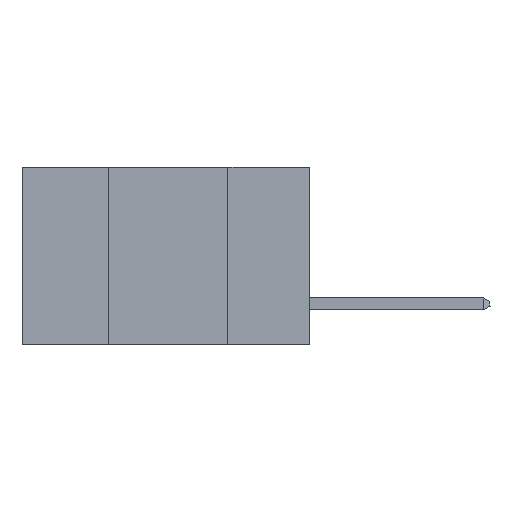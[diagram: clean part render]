
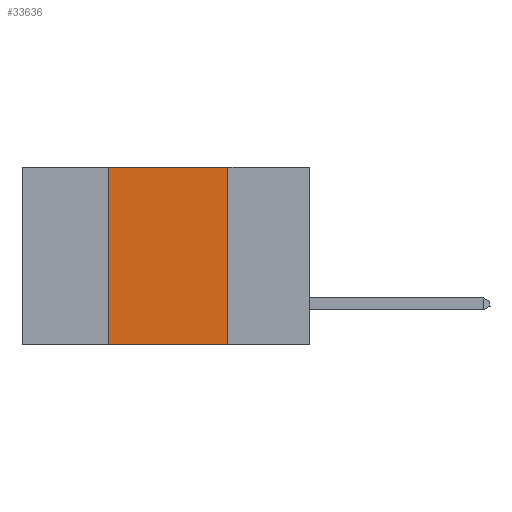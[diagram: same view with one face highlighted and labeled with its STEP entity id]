
A CAD part, left-side view. The second image highlights one B-rep face of the part: STEP entity #33636.
In plain terms, the highlighted planar face has unit normal (-1, 0, 0).
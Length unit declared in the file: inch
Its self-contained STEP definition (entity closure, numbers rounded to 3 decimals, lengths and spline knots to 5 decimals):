
#417 = ORIENTED_EDGE ( 'NONE', *, *, #23287, .F. ) ;
#500 = EDGE_CURVE ( 'NONE', #6923, #35511, #14397, .T. ) ;
#2125 = CARTESIAN_POINT ( 'NONE',  ( 0., 0.6, 0. ) ) ;
#2454 = VERTEX_POINT ( 'NONE', #45039 ) ;
#3004 = EDGE_LOOP ( 'NONE', ( #417, #21141, #40654, #37563 ) ) ;
#6719 = EDGE_CURVE ( 'NONE', #6923, #34437, #26632, .T. ) ;
#6923 = VERTEX_POINT ( 'NONE', #41657 ) ;
#8187 = CARTESIAN_POINT ( 'NONE',  ( 0., 0.6, -0.37 ) ) ;
#9260 = DIRECTION ( 'NONE',  ( 1., 0., 0. ) ) ;
#12655 = CARTESIAN_POINT ( 'NONE',  ( 0., 0.42, 0. ) ) ;
#13106 = DIRECTION ( 'NONE',  ( 0., 0., -1. ) ) ;
#13385 = FACE_OUTER_BOUND ( 'NONE', #3004, .T. ) ;
#14397 = LINE ( 'NONE', #8187, #44097 ) ;
#16595 = PLANE ( 'NONE',  #24044 ) ;
#16875 = EDGE_CURVE ( 'NONE', #34437, #2454, #33402, .T. ) ;
#20371 = CARTESIAN_POINT ( 'NONE',  ( 0., 0.17, 0. ) ) ;
#21027 = DIRECTION ( 'NONE',  ( 0., 0., -1. ) ) ;
#21141 = ORIENTED_EDGE ( 'NONE', *, *, #16875, .F. ) ;
#22989 = DIRECTION ( 'NONE',  ( 0., -1., 0. ) ) ;
#23287 = EDGE_CURVE ( 'NONE', #2454, #35511, #37252, .T. ) ;
#24044 = AXIS2_PLACEMENT_3D ( 'NONE', #2125, #9260, #13106 ) ;
#26156 = CARTESIAN_POINT ( 'NONE',  ( 0., 0.17, -0.37 ) ) ;
#26632 = LINE ( 'NONE', #39407, #32417 ) ;
#26880 = DIRECTION ( 'NONE',  ( 0., -1., 0. ) ) ;
#30858 = CARTESIAN_POINT ( 'NONE',  ( 0., 0.6, 0. ) ) ;
#32195 = DIRECTION ( 'NONE',  ( 0., 0., 1. ) ) ;
#32315 = VECTOR ( 'NONE', #26880, 39.37008 ) ;
#32417 = VECTOR ( 'NONE', #32195, 39.37008 ) ;
#33402 = LINE ( 'NONE', #30858, #32315 ) ;
#33636 = ADVANCED_FACE ( 'NONE', ( #13385 ), #16595, .F. ) ;
#34374 = VECTOR ( 'NONE', #21027, 39.37008 ) ;
#34437 = VERTEX_POINT ( 'NONE', #12655 ) ;
#35511 = VERTEX_POINT ( 'NONE', #26156 ) ;
#37252 = LINE ( 'NONE', #20371, #34374 ) ;
#37563 = ORIENTED_EDGE ( 'NONE', *, *, #500, .T. ) ;
#39407 = CARTESIAN_POINT ( 'NONE',  ( 0., 0.42, 0. ) ) ;
#40654 = ORIENTED_EDGE ( 'NONE', *, *, #6719, .F. ) ;
#41657 = CARTESIAN_POINT ( 'NONE',  ( 0., 0.42, -0.37 ) ) ;
#44097 = VECTOR ( 'NONE', #22989, 39.37008 ) ;
#45039 = CARTESIAN_POINT ( 'NONE',  ( 0., 0.17, 0. ) ) ;
